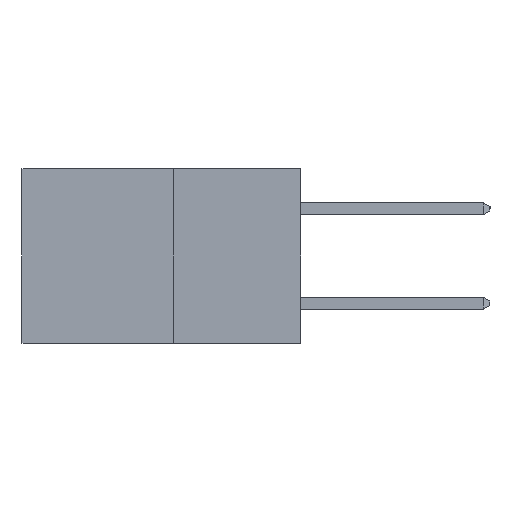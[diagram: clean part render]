
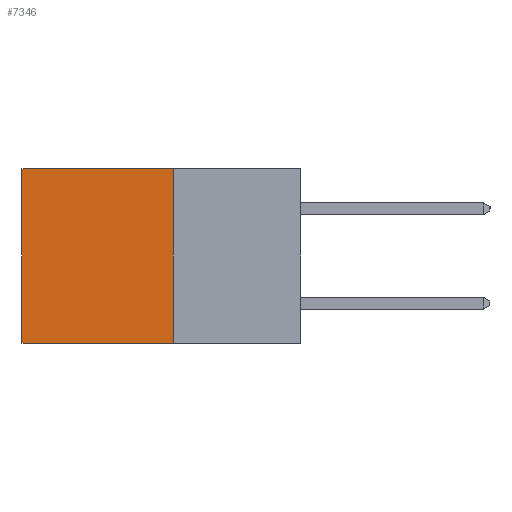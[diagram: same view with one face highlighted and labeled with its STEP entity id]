
A CAD part, left-side view. The second image highlights one B-rep face of the part: STEP entity #7346.
In plain terms, the highlighted planar face has unit normal (-1, 0, 0).
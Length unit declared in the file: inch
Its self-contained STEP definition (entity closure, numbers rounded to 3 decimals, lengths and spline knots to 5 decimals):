
#31 = VERTEX_POINT ( 'NONE', #3850 ) ;
#961 = VERTEX_POINT ( 'NONE', #5349 ) ;
#2060 = VERTEX_POINT ( 'NONE', #5600 ) ;
#2728 = CARTESIAN_POINT ( 'NONE',  ( 0.277, 0.27, 0. ) ) ;
#2841 = DIRECTION ( 'NONE',  ( 0., 1., 0. ) ) ;
#2905 = DIRECTION ( 'NONE',  ( 0., 1., 0. ) ) ;
#3850 = CARTESIAN_POINT ( 'NONE',  ( 0.277, 0.27, -0.37 ) ) ;
#4116 = DIRECTION ( 'NONE',  ( 0., 0., -1. ) ) ;
#4237 = CARTESIAN_POINT ( 'NONE',  ( 0.277, 0.59, -0.37 ) ) ;
#4475 = CARTESIAN_POINT ( 'NONE',  ( 0.277, 0.27, -0.37 ) ) ;
#4495 = VECTOR ( 'NONE', #2905, 39.37008 ) ;
#4601 = EDGE_CURVE ( 'NONE', #8847, #2060, #5850, .T. ) ;
#5349 = CARTESIAN_POINT ( 'NONE',  ( 0.277, 0.59, -0.37 ) ) ;
#5440 = FACE_OUTER_BOUND ( 'NONE', #8084, .T. ) ;
#5600 = CARTESIAN_POINT ( 'NONE',  ( 0.277, 0.59, 0. ) ) ;
#5850 = LINE ( 'NONE', #2728, #9379 ) ;
#5917 = EDGE_CURVE ( 'NONE', #8847, #31, #6168, .T. ) ;
#5959 = ORIENTED_EDGE ( 'NONE', *, *, #8951, .T. ) ;
#6168 = LINE ( 'NONE', #7150, #6393 ) ;
#6211 = LINE ( 'NONE', #4475, #4495 ) ;
#6393 = VECTOR ( 'NONE', #7510, 39.37008 ) ;
#6634 = CARTESIAN_POINT ( 'NONE',  ( 0.277, 0.27, 0. ) ) ;
#6750 = ORIENTED_EDGE ( 'NONE', *, *, #9345, .F. ) ;
#6894 = DIRECTION ( 'NONE',  ( 0., 0., -1. ) ) ;
#6905 = DIRECTION ( 'NONE',  ( 1., 0., 0. ) ) ;
#6916 = PLANE ( 'NONE',  #8714 ) ;
#6936 = CARTESIAN_POINT ( 'NONE',  ( 0.277, 0.27, -0.37 ) ) ;
#6997 = ORIENTED_EDGE ( 'NONE', *, *, #5917, .F. ) ;
#7150 = CARTESIAN_POINT ( 'NONE',  ( 0.277, 0.27, -0.37 ) ) ;
#7346 = ADVANCED_FACE ( 'NONE', ( #5440 ), #6916, .F. ) ;
#7510 = DIRECTION ( 'NONE',  ( 0., 0., -1. ) ) ;
#7652 = ORIENTED_EDGE ( 'NONE', *, *, #4601, .T. ) ;
#7893 = VECTOR ( 'NONE', #4116, 39.37008 ) ;
#8084 = EDGE_LOOP ( 'NONE', ( #5959, #6750, #6997, #7652 ) ) ;
#8344 = LINE ( 'NONE', #4237, #7893 ) ;
#8714 = AXIS2_PLACEMENT_3D ( 'NONE', #6936, #6905, #6894 ) ;
#8847 = VERTEX_POINT ( 'NONE', #6634 ) ;
#8951 = EDGE_CURVE ( 'NONE', #2060, #961, #8344, .T. ) ;
#9345 = EDGE_CURVE ( 'NONE', #31, #961, #6211, .T. ) ;
#9379 = VECTOR ( 'NONE', #2841, 39.37008 ) ;
